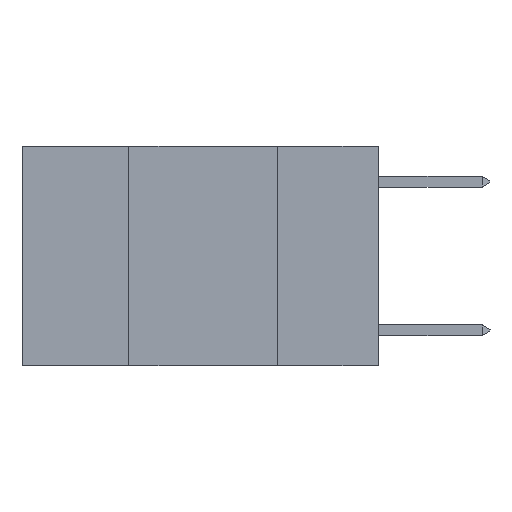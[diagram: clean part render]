
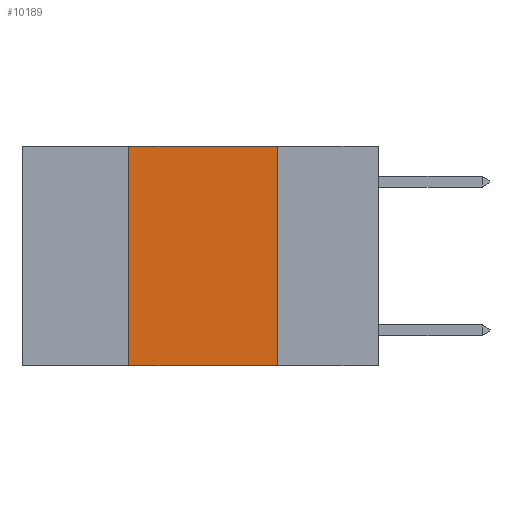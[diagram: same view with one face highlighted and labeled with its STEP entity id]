
A CAD part, left-side view. The second image highlights one B-rep face of the part: STEP entity #10189.
In plain terms, the highlighted planar face has unit normal (-1, 0, 0).
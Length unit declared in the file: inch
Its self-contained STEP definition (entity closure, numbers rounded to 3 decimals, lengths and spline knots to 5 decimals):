
#848 = VERTEX_POINT ( 'NONE', #10940 ) ;
#901 = EDGE_LOOP ( 'NONE', ( #7072, #7520, #9410, #11519 ) ) ;
#1125 = EDGE_CURVE ( 'NONE', #6472, #6640, #9336, .T. ) ;
#1479 = VERTEX_POINT ( 'NONE', #4958 ) ;
#1717 = DIRECTION ( 'NONE',  ( 0., -1., 0. ) ) ;
#1969 = PLANE ( 'NONE',  #8972 ) ;
#3378 = LINE ( 'NONE', #7225, #9954 ) ;
#3779 = CARTESIAN_POINT ( 'NONE',  ( 0., 0.6, 0. ) ) ;
#3871 = EDGE_CURVE ( 'NONE', #6472, #848, #3378, .T. ) ;
#4584 = VECTOR ( 'NONE', #6255, 39.37008 ) ;
#4686 = CARTESIAN_POINT ( 'NONE',  ( 0., 0.42, -0.37 ) ) ;
#4694 = DIRECTION ( 'NONE',  ( 0., 0., -1. ) ) ;
#4700 = EDGE_CURVE ( 'NONE', #1479, #848, #7399, .T. ) ;
#4924 = VECTOR ( 'NONE', #6959, 39.37008 ) ;
#4958 = CARTESIAN_POINT ( 'NONE',  ( 0., 0.17, 0. ) ) ;
#5277 = CARTESIAN_POINT ( 'NONE',  ( 0., 0.42, 0. ) ) ;
#5910 = CARTESIAN_POINT ( 'NONE',  ( 0., 0.42, 0. ) ) ;
#6255 = DIRECTION ( 'NONE',  ( 0., 0., 1. ) ) ;
#6288 = CARTESIAN_POINT ( 'NONE',  ( 0., 0.6, 0. ) ) ;
#6472 = VERTEX_POINT ( 'NONE', #4686 ) ;
#6640 = VERTEX_POINT ( 'NONE', #5910 ) ;
#6892 = LINE ( 'NONE', #6288, #9451 ) ;
#6959 = DIRECTION ( 'NONE',  ( 0., 0., -1. ) ) ;
#7000 = FACE_OUTER_BOUND ( 'NONE', #901, .T. ) ;
#7072 = ORIENTED_EDGE ( 'NONE', *, *, #4700, .F. ) ;
#7225 = CARTESIAN_POINT ( 'NONE',  ( 0., 0.6, -0.37 ) ) ;
#7399 = LINE ( 'NONE', #10335, #4924 ) ;
#7520 = ORIENTED_EDGE ( 'NONE', *, *, #8875, .F. ) ;
#8875 = EDGE_CURVE ( 'NONE', #6640, #1479, #6892, .T. ) ;
#8949 = DIRECTION ( 'NONE',  ( 0., -1., 0. ) ) ;
#8972 = AXIS2_PLACEMENT_3D ( 'NONE', #3779, #10028, #4694 ) ;
#9336 = LINE ( 'NONE', #5277, #4584 ) ;
#9410 = ORIENTED_EDGE ( 'NONE', *, *, #1125, .F. ) ;
#9451 = VECTOR ( 'NONE', #1717, 39.37008 ) ;
#9954 = VECTOR ( 'NONE', #8949, 39.37008 ) ;
#10028 = DIRECTION ( 'NONE',  ( 1., 0., 0. ) ) ;
#10189 = ADVANCED_FACE ( 'NONE', ( #7000 ), #1969, .F. ) ;
#10335 = CARTESIAN_POINT ( 'NONE',  ( 0., 0.17, 0. ) ) ;
#10940 = CARTESIAN_POINT ( 'NONE',  ( 0., 0.17, -0.37 ) ) ;
#11519 = ORIENTED_EDGE ( 'NONE', *, *, #3871, .T. ) ;
